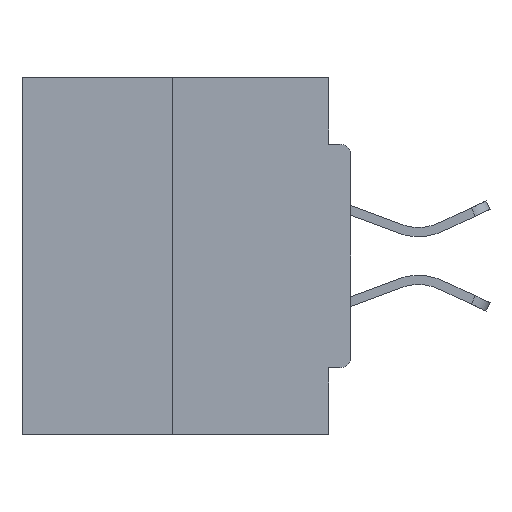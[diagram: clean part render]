
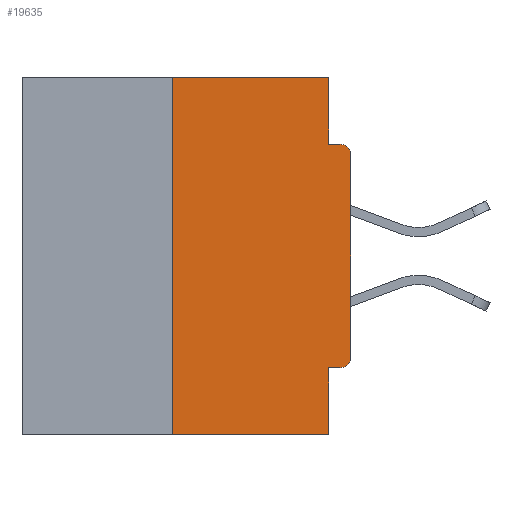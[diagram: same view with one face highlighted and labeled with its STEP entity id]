
A CAD part, left-side view. The second image highlights one B-rep face of the part: STEP entity #19635.
In plain terms, the highlighted planar face has unit normal (-1, 0, 0).
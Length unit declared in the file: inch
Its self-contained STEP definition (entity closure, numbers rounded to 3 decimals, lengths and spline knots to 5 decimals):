
#104 = DIRECTION ( 'NONE',  ( 0., -1., 0. ) ) ;
#185 = DIRECTION ( 'NONE',  ( -1., 0., 0. ) ) ;
#196 = VERTEX_POINT ( 'NONE', #35311 ) ;
#214 = LINE ( 'NONE', #5273, #19604 ) ;
#284 = CARTESIAN_POINT ( 'NONE',  ( 0., 0.015, -0.0935 ) ) ;
#373 = LINE ( 'NONE', #19084, #19267 ) ;
#629 = CARTESIAN_POINT ( 'NONE',  ( 0., 0.031, -0.0935 ) ) ;
#1003 = EDGE_CURVE ( 'NONE', #1934, #33447, #214, .T. ) ;
#1781 = EDGE_CURVE ( 'NONE', #33447, #9092, #28324, .T. ) ;
#1788 = LINE ( 'NONE', #9921, #8384 ) ;
#1934 = VERTEX_POINT ( 'NONE', #17571 ) ;
#2214 = DIRECTION ( 'NONE',  ( 0., -1., 0. ) ) ;
#2564 = DIRECTION ( 'NONE',  ( 0., 0., 1. ) ) ;
#4107 = AXIS2_PLACEMENT_3D ( 'NONE', #22609, #8226, #14789 ) ;
#4249 = ORIENTED_EDGE ( 'NONE', *, *, #1003, .T. ) ;
#4400 = VERTEX_POINT ( 'NONE', #26436 ) ;
#5273 = CARTESIAN_POINT ( 'NONE',  ( 0., 0., 0. ) ) ;
#5300 = EDGE_CURVE ( 'NONE', #19184, #6879, #17026, .T. ) ;
#5324 = EDGE_LOOP ( 'NONE', ( #17014, #16213, #7968, #9317, #11441, #30563, #4249, #20447, #15795, #30062 ) ) ;
#5753 = AXIS2_PLACEMENT_3D ( 'NONE', #25819, #185, #25594 ) ;
#6879 = VERTEX_POINT ( 'NONE', #17463 ) ;
#7718 = VECTOR ( 'NONE', #104, 39.37008 ) ;
#7792 = DIRECTION ( 'NONE',  ( 0., 0., -1. ) ) ;
#7873 = DIRECTION ( 'NONE',  ( 0., 0., 1. ) ) ;
#7879 = DIRECTION ( 'NONE',  ( 0., 0., -1. ) ) ;
#7968 = ORIENTED_EDGE ( 'NONE', *, *, #29843, .T. ) ;
#8226 = DIRECTION ( 'NONE',  ( 1., 0., 0. ) ) ;
#8384 = VECTOR ( 'NONE', #24064, 39.37008 ) ;
#9092 = VERTEX_POINT ( 'NONE', #284 ) ;
#9317 = ORIENTED_EDGE ( 'NONE', *, *, #15154, .F. ) ;
#9445 = FACE_OUTER_BOUND ( 'NONE', #5324, .T. ) ;
#9830 = VECTOR ( 'NONE', #7873, 39.37008 ) ;
#9921 = CARTESIAN_POINT ( 'NONE',  ( 0., 0., -0.4065 ) ) ;
#10345 = CARTESIAN_POINT ( 'NONE',  ( 0., 0.25, 0. ) ) ;
#11441 = ORIENTED_EDGE ( 'NONE', *, *, #24020, .F. ) ;
#11640 = LINE ( 'NONE', #26175, #27943 ) ;
#13242 = CARTESIAN_POINT ( 'NONE',  ( 0., 0.031, -0.5 ) ) ;
#13764 = VERTEX_POINT ( 'NONE', #629 ) ;
#14148 = EDGE_CURVE ( 'NONE', #34123, #1934, #33663, .T. ) ;
#14342 = VERTEX_POINT ( 'NONE', #28114 ) ;
#14789 = DIRECTION ( 'NONE',  ( 0., 0., -1. ) ) ;
#15154 = EDGE_CURVE ( 'NONE', #14342, #4400, #24729, .T. ) ;
#15795 = ORIENTED_EDGE ( 'NONE', *, *, #23361, .F. ) ;
#16213 = ORIENTED_EDGE ( 'NONE', *, *, #26815, .F. ) ;
#17014 = ORIENTED_EDGE ( 'NONE', *, *, #5300, .F. ) ;
#17026 = LINE ( 'NONE', #25626, #7718 ) ;
#17463 = CARTESIAN_POINT ( 'NONE',  ( 0., 0.031, 0. ) ) ;
#17571 = CARTESIAN_POINT ( 'NONE',  ( 0., 0., -0.3915 ) ) ;
#18821 = CARTESIAN_POINT ( 'NONE',  ( 0., 0., -0.1085 ) ) ;
#19084 = CARTESIAN_POINT ( 'NONE',  ( 0., 0.46, -0.5 ) ) ;
#19184 = VERTEX_POINT ( 'NONE', #10345 ) ;
#19267 = VECTOR ( 'NONE', #2214, 39.37008 ) ;
#19604 = VECTOR ( 'NONE', #2564, 39.37008 ) ;
#19635 = ADVANCED_FACE ( 'NONE', ( #9445 ), #33763, .F. ) ;
#20354 = DIRECTION ( 'NONE',  ( 0., 0., -1. ) ) ;
#20447 = ORIENTED_EDGE ( 'NONE', *, *, #1781, .T. ) ;
#20777 = LINE ( 'NONE', #27473, #27854 ) ;
#21769 = DIRECTION ( 'NONE',  ( -1., 0., 0. ) ) ;
#22609 = CARTESIAN_POINT ( 'NONE',  ( 0., 0.46, 0. ) ) ;
#23361 = EDGE_CURVE ( 'NONE', #13764, #9092, #20777, .T. ) ;
#24020 = EDGE_CURVE ( 'NONE', #34123, #14342, #1788, .T. ) ;
#24064 = DIRECTION ( 'NONE',  ( 0., 1., 0. ) ) ;
#24619 = DIRECTION ( 'NONE',  ( 0., -1., 0. ) ) ;
#24729 = LINE ( 'NONE', #13242, #34005 ) ;
#24754 = CARTESIAN_POINT ( 'NONE',  ( 0., 0.25, 0. ) ) ;
#25594 = DIRECTION ( 'NONE',  ( 0., 0., -1. ) ) ;
#25626 = CARTESIAN_POINT ( 'NONE',  ( 0., 0.46, 0. ) ) ;
#25819 = CARTESIAN_POINT ( 'NONE',  ( 0., 0.015, -0.1085 ) ) ;
#26175 = CARTESIAN_POINT ( 'NONE',  ( 0., 0.031, 0. ) ) ;
#26317 = EDGE_CURVE ( 'NONE', #6879, #13764, #11640, .T. ) ;
#26436 = CARTESIAN_POINT ( 'NONE',  ( 0., 0.031, -0.5 ) ) ;
#26815 = EDGE_CURVE ( 'NONE', #196, #19184, #31456, .T. ) ;
#27473 = CARTESIAN_POINT ( 'NONE',  ( 0., 0., -0.0935 ) ) ;
#27854 = VECTOR ( 'NONE', #24619, 39.37008 ) ;
#27943 = VECTOR ( 'NONE', #20354, 39.37008 ) ;
#28114 = CARTESIAN_POINT ( 'NONE',  ( 0., 0.031, -0.4065 ) ) ;
#28324 = CIRCLE ( 'NONE', #5753, 0.015 ) ;
#29843 = EDGE_CURVE ( 'NONE', #196, #4400, #373, .T. ) ;
#29984 = AXIS2_PLACEMENT_3D ( 'NONE', #33154, #21769, #7879 ) ;
#30062 = ORIENTED_EDGE ( 'NONE', *, *, #26317, .F. ) ;
#30563 = ORIENTED_EDGE ( 'NONE', *, *, #14148, .T. ) ;
#31456 = LINE ( 'NONE', #24754, #9830 ) ;
#33154 = CARTESIAN_POINT ( 'NONE',  ( 0., 0.015, -0.3915 ) ) ;
#33447 = VERTEX_POINT ( 'NONE', #18821 ) ;
#33663 = CIRCLE ( 'NONE', #29984, 0.015 ) ;
#33763 = PLANE ( 'NONE',  #4107 ) ;
#34005 = VECTOR ( 'NONE', #7792, 39.37008 ) ;
#34123 = VERTEX_POINT ( 'NONE', #36512 ) ;
#35311 = CARTESIAN_POINT ( 'NONE',  ( 0., 0.25, -0.5 ) ) ;
#36512 = CARTESIAN_POINT ( 'NONE',  ( 0., 0.015, -0.4065 ) ) ;
